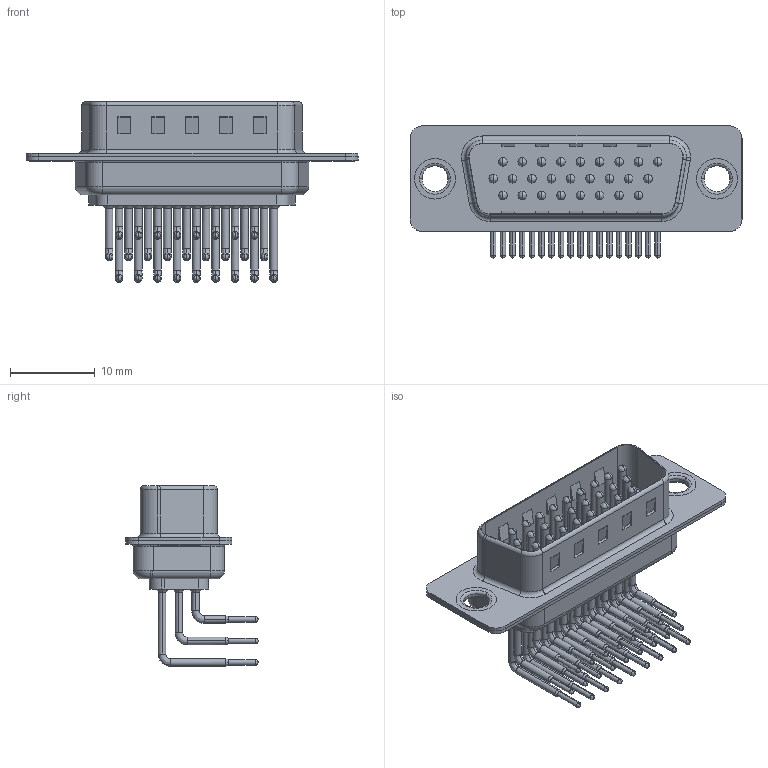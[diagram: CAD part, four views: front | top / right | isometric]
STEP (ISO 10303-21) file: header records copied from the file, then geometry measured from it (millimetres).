
FILE_DESCRIPTION (( 'STEP AP203' ), '1' );
FILE_NAME ('633-M26-363-WN1.STEP', '2018-09-27T23:14:42', ( '' ), ( '' ), 'SwSTEP 2.0', 'SolidWorks 2016', '' );
FILE_SCHEMA (( 'CONFIG_CONTROL_DESIGN' ));
Length unit declared in the file: millimetre
Products named in the file (8): 633M Shell Front_26 Contacts; 633M Shell Rear_26 Contacts; 633M Contact Row 1; 633M Contact Row 2; 633M Contact Row 3; 633M Thru Hole Rivet; 633-M26-363-WN1; 633M Housing_26 Contacts
Assembly tree (31 placements, depth 2):
  633-M26-363-WN1
    633M Housing_26 Contacts
    633M Shell Front_26 Contacts
    633M Shell Rear_26 Contacts
    633M Contact Row 1  x9
    633M Contact Row 2  x9
    633M Contact Row 3  x8
    633M Thru Hole Rivet  x2
Bounding box: 39.2 x 15.6 x 21.32 mm (x, y, z)
Volume: 2011.5 mm3; surface area: 6546 mm2
Topology: 31 solids, 31 shells, 3174 faces, 8853 edges, 5752 vertices
Faces by surface type: plane 1803, cylinder 1053, bspline 156, cone 104, torus 58
Entity records: 26640 total; most frequent: CARTESIAN_POINT 4587, DIRECTION 4523, ORIENTED_EDGE 4138, EDGE_CURVE 2069, AXIS2_PLACEMENT_3D 1645, VERTEX_POINT 1342, LINE 1233, VECTOR 1233
